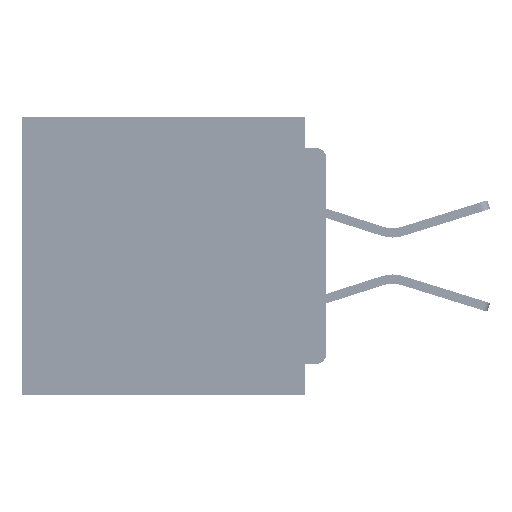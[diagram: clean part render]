
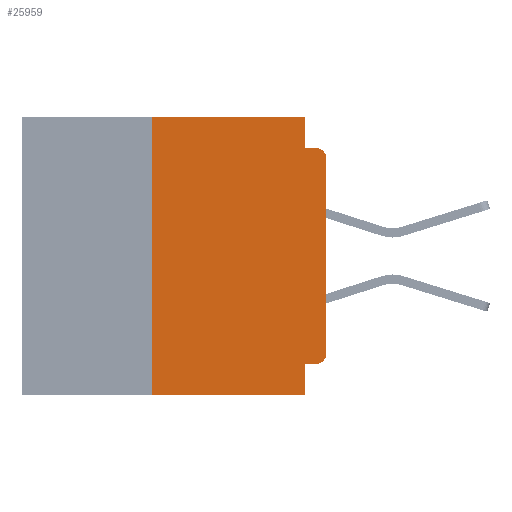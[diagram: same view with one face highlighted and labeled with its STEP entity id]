
A CAD part, left-side view. The second image highlights one B-rep face of the part: STEP entity #25959.
In plain terms, the highlighted planar face has unit normal (-1, 0, 0).
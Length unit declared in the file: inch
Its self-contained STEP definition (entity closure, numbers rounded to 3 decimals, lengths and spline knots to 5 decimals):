
#2467 = LINE ( 'NONE', #38139, #26446 ) ;
#2803 = VECTOR ( 'NONE', #43660, 39.37008 ) ;
#3160 = VERTEX_POINT ( 'NONE', #32159 ) ;
#3865 = CARTESIAN_POINT ( 'NONE',  ( 0., 0.031, 0. ) ) ;
#4288 = DIRECTION ( 'NONE',  ( 0., 0., -1. ) ) ;
#4526 = LINE ( 'NONE', #21626, #2803 ) ;
#6754 = EDGE_CURVE ( 'NONE', #53120, #60714, #22366, .T. ) ;
#8838 = EDGE_CURVE ( 'NONE', #24233, #30461, #32713, .T. ) ;
#9978 = CARTESIAN_POINT ( 'NONE',  ( 0., 0.25, -0.4 ) ) ;
#10119 = CARTESIAN_POINT ( 'NONE',  ( 0., 0., -0.355 ) ) ;
#10149 = ORIENTED_EDGE ( 'NONE', *, *, #52079, .F. ) ;
#10352 = ORIENTED_EDGE ( 'NONE', *, *, #61595, .T. ) ;
#11338 = ORIENTED_EDGE ( 'NONE', *, *, #28112, .F. ) ;
#12392 = DIRECTION ( 'NONE',  ( 0., -1., 0. ) ) ;
#12803 = CARTESIAN_POINT ( 'NONE',  ( 0., 0.031, -0.045 ) ) ;
#12875 = CARTESIAN_POINT ( 'NONE',  ( 0., 0.437, 0. ) ) ;
#13968 = CARTESIAN_POINT ( 'NONE',  ( 0., 0.031, -0.4 ) ) ;
#14903 = ORIENTED_EDGE ( 'NONE', *, *, #38475, .F. ) ;
#15006 = VERTEX_POINT ( 'NONE', #13968 ) ;
#15077 = DIRECTION ( 'NONE',  ( 1., 0., 0. ) ) ;
#15368 = DIRECTION ( 'NONE',  ( 0., 0., -1. ) ) ;
#16278 = CARTESIAN_POINT ( 'NONE',  ( 0., 0.015, -0.34 ) ) ;
#16298 = CARTESIAN_POINT ( 'NONE',  ( 0., 0., -0.06 ) ) ;
#19360 = VERTEX_POINT ( 'NONE', #25071 ) ;
#21626 = CARTESIAN_POINT ( 'NONE',  ( 0., 0., 0. ) ) ;
#21726 = DIRECTION ( 'NONE',  ( 0., 0., -1. ) ) ;
#21729 = VERTEX_POINT ( 'NONE', #60975 ) ;
#21842 = VERTEX_POINT ( 'NONE', #12803 ) ;
#21867 = ORIENTED_EDGE ( 'NONE', *, *, #6754, .F. ) ;
#22366 = LINE ( 'NONE', #10119, #49762 ) ;
#23171 = LINE ( 'NONE', #12875, #36013 ) ;
#23545 = FACE_OUTER_BOUND ( 'NONE', #61831, .T. ) ;
#23869 = ORIENTED_EDGE ( 'NONE', *, *, #70745, .F. ) ;
#24041 = LINE ( 'NONE', #9978, #51401 ) ;
#24233 = VERTEX_POINT ( 'NONE', #16298 ) ;
#25071 = CARTESIAN_POINT ( 'NONE',  ( 0., 0., -0.34 ) ) ;
#25461 = AXIS2_PLACEMENT_3D ( 'NONE', #16278, #54486, #21726 ) ;
#25959 = ADVANCED_FACE ( 'NONE', ( #23545 ), #37039, .F. ) ;
#26446 = VECTOR ( 'NONE', #54603, 39.37008 ) ;
#26595 = DIRECTION ( 'NONE',  ( 0., 1., 0. ) ) ;
#27779 = DIRECTION ( 'NONE',  ( -1., 0., 0. ) ) ;
#28033 = CARTESIAN_POINT ( 'NONE',  ( 0., 0.437, -0.4 ) ) ;
#28112 = EDGE_CURVE ( 'NONE', #21729, #44516, #24041, .T. ) ;
#28957 = EDGE_CURVE ( 'NONE', #21729, #15006, #40201, .T. ) ;
#30461 = VERTEX_POINT ( 'NONE', #54465 ) ;
#31351 = AXIS2_PLACEMENT_3D ( 'NONE', #31595, #15077, #4288 ) ;
#31595 = CARTESIAN_POINT ( 'NONE',  ( 0., 0.437, 0. ) ) ;
#32159 = CARTESIAN_POINT ( 'NONE',  ( 0., 0.031, 0. ) ) ;
#32713 = CIRCLE ( 'NONE', #51550, 0.015 ) ;
#33671 = ORIENTED_EDGE ( 'NONE', *, *, #70435, .T. ) ;
#33909 = CIRCLE ( 'NONE', #25461, 0.015 ) ;
#36013 = VECTOR ( 'NONE', #12392, 39.37008 ) ;
#37039 = PLANE ( 'NONE',  #31351 ) ;
#38139 = CARTESIAN_POINT ( 'NONE',  ( 0., 0., -0.045 ) ) ;
#38475 = EDGE_CURVE ( 'NONE', #44516, #3160, #23171, .T. ) ;
#39035 = DIRECTION ( 'NONE',  ( 0., -1., 0. ) ) ;
#40201 = LINE ( 'NONE', #28033, #67399 ) ;
#43660 = DIRECTION ( 'NONE',  ( 0., 0., 1. ) ) ;
#43937 = VECTOR ( 'NONE', #15368, 39.37008 ) ;
#44516 = VERTEX_POINT ( 'NONE', #61025 ) ;
#49762 = VECTOR ( 'NONE', #26595, 39.37008 ) ;
#51401 = VECTOR ( 'NONE', #53679, 39.37008 ) ;
#51550 = AXIS2_PLACEMENT_3D ( 'NONE', #60448, #27779, #65892 ) ;
#52079 = EDGE_CURVE ( 'NONE', #60714, #15006, #58406, .T. ) ;
#52729 = CARTESIAN_POINT ( 'NONE',  ( 0., 0.015, -0.355 ) ) ;
#53120 = VERTEX_POINT ( 'NONE', #52729 ) ;
#53562 = CARTESIAN_POINT ( 'NONE',  ( 0., 0.031, -0.4 ) ) ;
#53679 = DIRECTION ( 'NONE',  ( 0., 0., 1. ) ) ;
#54465 = CARTESIAN_POINT ( 'NONE',  ( 0., 0.015, -0.045 ) ) ;
#54486 = DIRECTION ( 'NONE',  ( -1., 0., 0. ) ) ;
#54513 = ORIENTED_EDGE ( 'NONE', *, *, #8838, .T. ) ;
#54603 = DIRECTION ( 'NONE',  ( 0., -1., 0. ) ) ;
#55186 = LINE ( 'NONE', #3865, #67910 ) ;
#58288 = CARTESIAN_POINT ( 'NONE',  ( 0., 0.031, -0.355 ) ) ;
#58406 = LINE ( 'NONE', #53562, #43937 ) ;
#58428 = ORIENTED_EDGE ( 'NONE', *, *, #28957, .T. ) ;
#58562 = DIRECTION ( 'NONE',  ( 0., 0., -1. ) ) ;
#60448 = CARTESIAN_POINT ( 'NONE',  ( 0., 0.015, -0.06 ) ) ;
#60714 = VERTEX_POINT ( 'NONE', #58288 ) ;
#60975 = CARTESIAN_POINT ( 'NONE',  ( 0., 0.25, -0.4 ) ) ;
#61025 = CARTESIAN_POINT ( 'NONE',  ( 0., 0.25, 0. ) ) ;
#61595 = EDGE_CURVE ( 'NONE', #19360, #24233, #4526, .T. ) ;
#61831 = EDGE_LOOP ( 'NONE', ( #10352, #54513, #65883, #23869, #14903, #11338, #58428, #10149, #21867, #33671 ) ) ;
#64089 = EDGE_CURVE ( 'NONE', #21842, #30461, #2467, .T. ) ;
#65883 = ORIENTED_EDGE ( 'NONE', *, *, #64089, .F. ) ;
#65892 = DIRECTION ( 'NONE',  ( 0., 0., -1. ) ) ;
#67399 = VECTOR ( 'NONE', #39035, 39.37008 ) ;
#67910 = VECTOR ( 'NONE', #58562, 39.37008 ) ;
#70435 = EDGE_CURVE ( 'NONE', #53120, #19360, #33909, .T. ) ;
#70745 = EDGE_CURVE ( 'NONE', #3160, #21842, #55186, .T. ) ;
